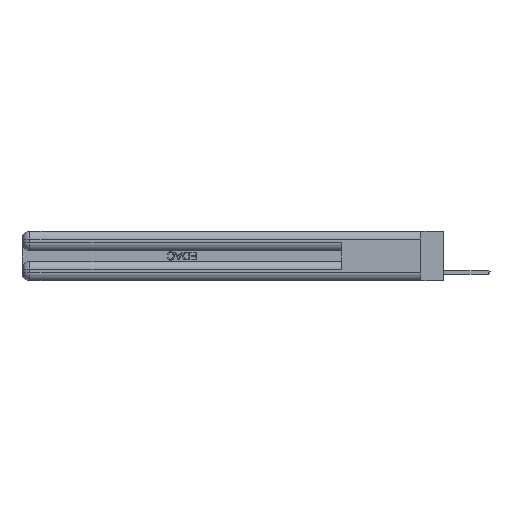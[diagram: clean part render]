
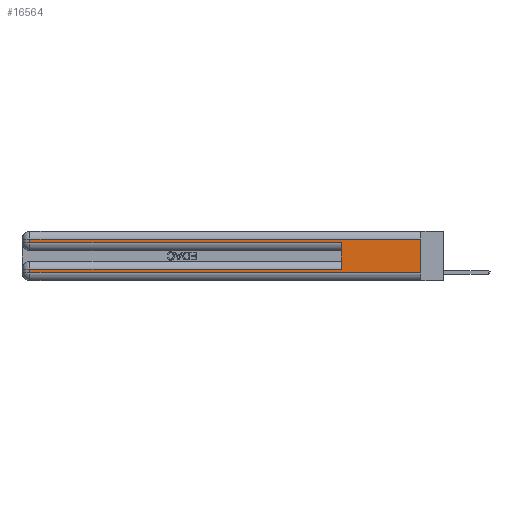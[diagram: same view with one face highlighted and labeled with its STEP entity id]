
A CAD part, left-side view. The second image highlights one B-rep face of the part: STEP entity #16564.
In plain terms, the highlighted planar face has unit normal (-1, 0, 0).
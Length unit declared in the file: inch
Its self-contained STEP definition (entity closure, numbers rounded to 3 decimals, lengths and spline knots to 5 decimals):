
#297 = CARTESIAN_POINT ( 'NONE',  ( 0., 0., 0.06 ) ) ;
#454 = VECTOR ( 'NONE', #13765, 39.37008 ) ;
#499 = LINE ( 'NONE', #26502, #18911 ) ;
#697 = CARTESIAN_POINT ( 'NONE',  ( 0., 0., 0.085 ) ) ;
#1375 = DIRECTION ( 'NONE',  ( 0., 0., 1. ) ) ;
#1489 = CARTESIAN_POINT ( 'NONE',  ( 0., 0.6, 0.145 ) ) ;
#1945 = LINE ( 'NONE', #1489, #20345 ) ;
#2537 = VERTEX_POINT ( 'NONE', #13501 ) ;
#3363 = EDGE_CURVE ( 'NONE', #2537, #24579, #19357, .T. ) ;
#3733 = VERTEX_POINT ( 'NONE', #6493 ) ;
#4005 = EDGE_CURVE ( 'NONE', #2537, #30561, #499, .T. ) ;
#4419 = VERTEX_POINT ( 'NONE', #33543 ) ;
#5324 = VECTOR ( 'NONE', #13794, 39.37008 ) ;
#5349 = ORIENTED_EDGE ( 'NONE', *, *, #12595, .F. ) ;
#5789 = ORIENTED_EDGE ( 'NONE', *, *, #3363, .F. ) ;
#6493 = CARTESIAN_POINT ( 'NONE',  ( 0., 0.6, 0.085 ) ) ;
#8209 = CARTESIAN_POINT ( 'NONE',  ( 0., 2.94, 0.06 ) ) ;
#8643 = ORIENTED_EDGE ( 'NONE', *, *, #14694, .T. ) ;
#9029 = DIRECTION ( 'NONE',  ( 0., 0., -1. ) ) ;
#9517 = VECTOR ( 'NONE', #15105, 39.37008 ) ;
#10827 = FACE_OUTER_BOUND ( 'NONE', #12339, .T. ) ;
#11002 = DIRECTION ( 'NONE',  ( 0., 1., 0. ) ) ;
#12057 = CARTESIAN_POINT ( 'NONE',  ( 0., 0., 0.37 ) ) ;
#12279 = ORIENTED_EDGE ( 'NONE', *, *, #15408, .T. ) ;
#12339 = EDGE_LOOP ( 'NONE', ( #5789, #32762, #17609, #8643, #5349, #21077, #12279, #26393 ) ) ;
#12595 = EDGE_CURVE ( 'NONE', #3733, #19090, #1945, .T. ) ;
#13501 = CARTESIAN_POINT ( 'NONE',  ( 0., 0., 0.31 ) ) ;
#13765 = DIRECTION ( 'NONE',  ( 0., -1., 0. ) ) ;
#13794 = DIRECTION ( 'NONE',  ( 0., 1., 0. ) ) ;
#14055 = VERTEX_POINT ( 'NONE', #16027 ) ;
#14128 = AXIS2_PLACEMENT_3D ( 'NONE', #16817, #29643, #9029 ) ;
#14350 = VECTOR ( 'NONE', #27086, 39.37008 ) ;
#14694 = EDGE_CURVE ( 'NONE', #14055, #19090, #27845, .T. ) ;
#15105 = DIRECTION ( 'NONE',  ( 0., 0., -1. ) ) ;
#15124 = VERTEX_POINT ( 'NONE', #8209 ) ;
#15408 = EDGE_CURVE ( 'NONE', #4419, #15124, #30718, .T. ) ;
#15814 = EDGE_CURVE ( 'NONE', #3733, #4419, #32725, .T. ) ;
#16027 = CARTESIAN_POINT ( 'NONE',  ( 0., 2.94, 0.285 ) ) ;
#16046 = DIRECTION ( 'NONE',  ( 0., -1., 0. ) ) ;
#16564 = ADVANCED_FACE ( 'NONE', ( #10827 ), #24359, .F. ) ;
#16817 = CARTESIAN_POINT ( 'NONE',  ( 0., 0., 0.37 ) ) ;
#17543 = CARTESIAN_POINT ( 'NONE',  ( 0., 0., 0.06 ) ) ;
#17609 = ORIENTED_EDGE ( 'NONE', *, *, #30762, .T. ) ;
#17923 = CARTESIAN_POINT ( 'NONE',  ( 0., 2.94, 0.31 ) ) ;
#18317 = CARTESIAN_POINT ( 'NONE',  ( 0., 0.6, 0.285 ) ) ;
#18382 = CARTESIAN_POINT ( 'NONE',  ( 0., 2.94, 0.37 ) ) ;
#18911 = VECTOR ( 'NONE', #11002, 39.37008 ) ;
#19090 = VERTEX_POINT ( 'NONE', #18317 ) ;
#19357 = LINE ( 'NONE', #12057, #9517 ) ;
#20242 = VECTOR ( 'NONE', #26344, 39.37008 ) ;
#20345 = VECTOR ( 'NONE', #1375, 39.37008 ) ;
#21077 = ORIENTED_EDGE ( 'NONE', *, *, #15814, .T. ) ;
#23479 = LINE ( 'NONE', #18382, #20242 ) ;
#24359 = PLANE ( 'NONE',  #14128 ) ;
#24579 = VERTEX_POINT ( 'NONE', #17543 ) ;
#24920 = LINE ( 'NONE', #297, #30249 ) ;
#26344 = DIRECTION ( 'NONE',  ( 0., 0., -1. ) ) ;
#26393 = ORIENTED_EDGE ( 'NONE', *, *, #29193, .T. ) ;
#26502 = CARTESIAN_POINT ( 'NONE',  ( 0., 0., 0.31 ) ) ;
#27086 = DIRECTION ( 'NONE',  ( 0., 0., -1. ) ) ;
#27845 = LINE ( 'NONE', #29440, #454 ) ;
#29177 = CARTESIAN_POINT ( 'NONE',  ( 0., 2.94, 0.37 ) ) ;
#29193 = EDGE_CURVE ( 'NONE', #15124, #24579, #24920, .T. ) ;
#29440 = CARTESIAN_POINT ( 'NONE',  ( 0., 0., 0.285 ) ) ;
#29643 = DIRECTION ( 'NONE',  ( 1., 0., 0. ) ) ;
#30249 = VECTOR ( 'NONE', #16046, 39.37008 ) ;
#30561 = VERTEX_POINT ( 'NONE', #17923 ) ;
#30718 = LINE ( 'NONE', #29177, #14350 ) ;
#30762 = EDGE_CURVE ( 'NONE', #30561, #14055, #23479, .T. ) ;
#32725 = LINE ( 'NONE', #697, #5324 ) ;
#32762 = ORIENTED_EDGE ( 'NONE', *, *, #4005, .T. ) ;
#33543 = CARTESIAN_POINT ( 'NONE',  ( 0., 2.94, 0.085 ) ) ;
